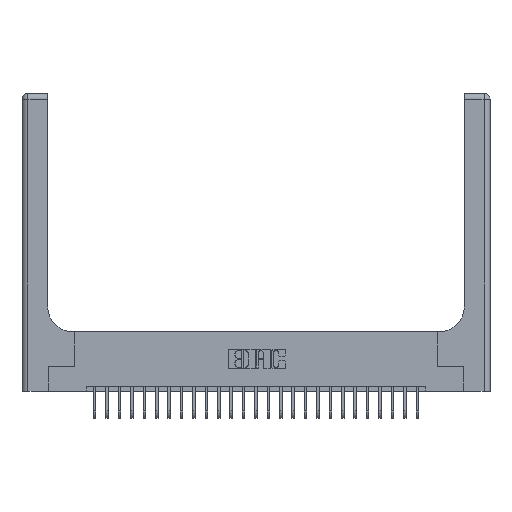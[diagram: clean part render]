
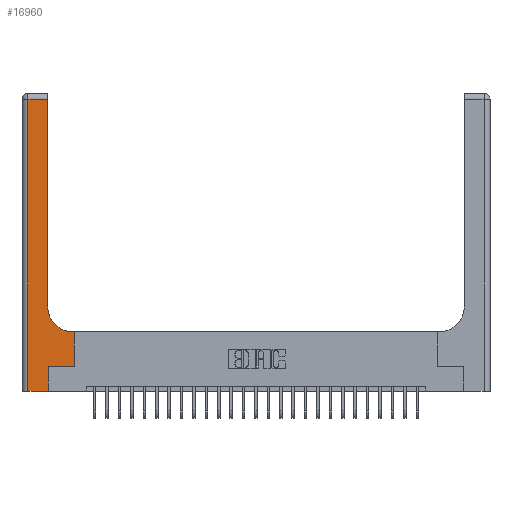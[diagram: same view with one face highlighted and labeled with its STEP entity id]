
A CAD part, top view. The second image highlights one B-rep face of the part: STEP entity #16960.
In plain terms, the highlighted planar face has unit normal (0, 0, 1).
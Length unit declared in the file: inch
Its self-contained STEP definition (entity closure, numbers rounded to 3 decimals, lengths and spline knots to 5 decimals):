
#190 = ORIENTED_EDGE ( 'NONE', *, *, #18022, .T. ) ;
#655 = VECTOR ( 'NONE', #13315, 39.37008 ) ;
#1040 = EDGE_LOOP ( 'NONE', ( #8527, #9706, #10069, #190, #14703, #18760, #19771, #19954, #10260 ) ) ;
#1065 = CARTESIAN_POINT ( 'NONE',  ( 0., 3., 0.37 ) ) ;
#2161 = EDGE_CURVE ( 'NONE', #21351, #19289, #5294, .T. ) ;
#2877 = DIRECTION ( 'NONE',  ( 1., 0., 0. ) ) ;
#2883 = EDGE_CURVE ( 'NONE', #23451, #7567, #9166, .T. ) ;
#2970 = CARTESIAN_POINT ( 'NONE',  ( 0.528, 0.25, 0.37 ) ) ;
#3231 = CARTESIAN_POINT ( 'NONE',  ( 0.528, 0.6, 0.37 ) ) ;
#3397 = LINE ( 'NONE', #18622, #20946 ) ;
#3525 = DIRECTION ( 'NONE',  ( 0., 1., 0. ) ) ;
#3604 = VERTEX_POINT ( 'NONE', #10961 ) ;
#3923 = CARTESIAN_POINT ( 'NONE',  ( 0.26, 0.6, 0.37 ) ) ;
#4763 = DIRECTION ( 'NONE',  ( 0., 0., -1. ) ) ;
#5294 = LINE ( 'NONE', #3923, #655 ) ;
#6018 = AXIS2_PLACEMENT_3D ( 'NONE', #8472, #4763, #2877 ) ;
#6460 = CARTESIAN_POINT ( 'NONE',  ( 0.06, 0., 0.37 ) ) ;
#7258 = EDGE_CURVE ( 'NONE', #19289, #13582, #13505, .T. ) ;
#7312 = LINE ( 'NONE', #11025, #17461 ) ;
#7535 = LINE ( 'NONE', #14578, #18467 ) ;
#7567 = VERTEX_POINT ( 'NONE', #18965 ) ;
#7776 = VECTOR ( 'NONE', #11744, 39.37008 ) ;
#7844 = EDGE_CURVE ( 'NONE', #7567, #14984, #7312, .T. ) ;
#8472 = CARTESIAN_POINT ( 'NONE',  ( 0.51, 0.85, 0.37 ) ) ;
#8489 = FACE_OUTER_BOUND ( 'NONE', #1040, .T. ) ;
#8527 = ORIENTED_EDGE ( 'NONE', *, *, #11330, .T. ) ;
#8617 = DIRECTION ( 'NONE',  ( -1., 0., 0. ) ) ;
#8698 = EDGE_CURVE ( 'NONE', #19963, #17725, #16502, .T. ) ;
#8926 = CARTESIAN_POINT ( 'NONE',  ( 0., 2.94, 0.37 ) ) ;
#9166 = LINE ( 'NONE', #8926, #13679 ) ;
#9706 = ORIENTED_EDGE ( 'NONE', *, *, #2883, .T. ) ;
#10069 = ORIENTED_EDGE ( 'NONE', *, *, #7844, .T. ) ;
#10260 = ORIENTED_EDGE ( 'NONE', *, *, #7258, .T. ) ;
#10961 = CARTESIAN_POINT ( 'NONE',  ( 0.265, 0., 0.37 ) ) ;
#11025 = CARTESIAN_POINT ( 'NONE',  ( 0.06, 3., 0.37 ) ) ;
#11330 = EDGE_CURVE ( 'NONE', #13582, #23451, #17827, .T. ) ;
#11744 = DIRECTION ( 'NONE',  ( 1., 0., 0. ) ) ;
#12366 = DIRECTION ( 'NONE',  ( -1., 0., 0. ) ) ;
#12445 = AXIS2_PLACEMENT_3D ( 'NONE', #1065, #24094, #8617 ) ;
#13315 = DIRECTION ( 'NONE',  ( -1., 0., 0. ) ) ;
#13505 = CIRCLE ( 'NONE', #6018, 0.25 ) ;
#13582 = VERTEX_POINT ( 'NONE', #17536 ) ;
#13586 = LINE ( 'NONE', #22778, #7776 ) ;
#13679 = VECTOR ( 'NONE', #12366, 39.37008 ) ;
#14363 = DIRECTION ( 'NONE',  ( 0., -1., 0. ) ) ;
#14578 = CARTESIAN_POINT ( 'NONE',  ( 0.265, 0., 0.37 ) ) ;
#14636 = CARTESIAN_POINT ( 'NONE',  ( 0.265, 0.25, 0.37 ) ) ;
#14703 = ORIENTED_EDGE ( 'NONE', *, *, #19427, .T. ) ;
#14984 = VERTEX_POINT ( 'NONE', #6460 ) ;
#15063 = DIRECTION ( 'NONE',  ( 0., 1., 0. ) ) ;
#15849 = CARTESIAN_POINT ( 'NONE',  ( 0.265, 0.25, 0.37 ) ) ;
#16502 = LINE ( 'NONE', #14636, #19607 ) ;
#16960 = ADVANCED_FACE ( 'NONE', ( #8489 ), #20234, .F. ) ;
#17087 = VECTOR ( 'NONE', #21795, 39.37008 ) ;
#17461 = VECTOR ( 'NONE', #14363, 39.37008 ) ;
#17536 = CARTESIAN_POINT ( 'NONE',  ( 0.26, 0.85, 0.37 ) ) ;
#17725 = VERTEX_POINT ( 'NONE', #2970 ) ;
#17827 = LINE ( 'NONE', #21914, #17087 ) ;
#18022 = EDGE_CURVE ( 'NONE', #14984, #3604, #13586, .T. ) ;
#18467 = VECTOR ( 'NONE', #15063, 39.37008 ) ;
#18622 = CARTESIAN_POINT ( 'NONE',  ( 0.528, 0.25, 0.37 ) ) ;
#18760 = ORIENTED_EDGE ( 'NONE', *, *, #8698, .T. ) ;
#18965 = CARTESIAN_POINT ( 'NONE',  ( 0.06, 2.94, 0.37 ) ) ;
#19289 = VERTEX_POINT ( 'NONE', #21772 ) ;
#19427 = EDGE_CURVE ( 'NONE', #3604, #19963, #7535, .T. ) ;
#19607 = VECTOR ( 'NONE', #22086, 39.37008 ) ;
#19771 = ORIENTED_EDGE ( 'NONE', *, *, #23466, .T. ) ;
#19954 = ORIENTED_EDGE ( 'NONE', *, *, #2161, .T. ) ;
#19963 = VERTEX_POINT ( 'NONE', #15849 ) ;
#20234 = PLANE ( 'NONE',  #12445 ) ;
#20946 = VECTOR ( 'NONE', #3525, 39.37008 ) ;
#21351 = VERTEX_POINT ( 'NONE', #3231 ) ;
#21772 = CARTESIAN_POINT ( 'NONE',  ( 0.51, 0.6, 0.37 ) ) ;
#21795 = DIRECTION ( 'NONE',  ( 0., 1., 0. ) ) ;
#21914 = CARTESIAN_POINT ( 'NONE',  ( 0.26, 3., 0.37 ) ) ;
#22086 = DIRECTION ( 'NONE',  ( 1., 0., 0. ) ) ;
#22778 = CARTESIAN_POINT ( 'NONE',  ( 0., 0., 0.37 ) ) ;
#23451 = VERTEX_POINT ( 'NONE', #23849 ) ;
#23466 = EDGE_CURVE ( 'NONE', #17725, #21351, #3397, .T. ) ;
#23849 = CARTESIAN_POINT ( 'NONE',  ( 0.26, 2.94, 0.37 ) ) ;
#24094 = DIRECTION ( 'NONE',  ( 0., 0., -1. ) ) ;
